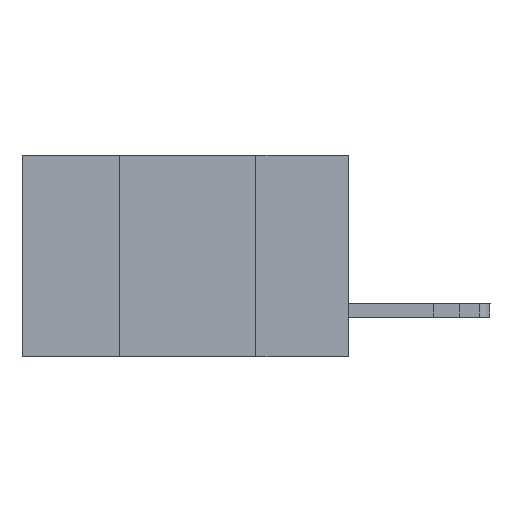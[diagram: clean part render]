
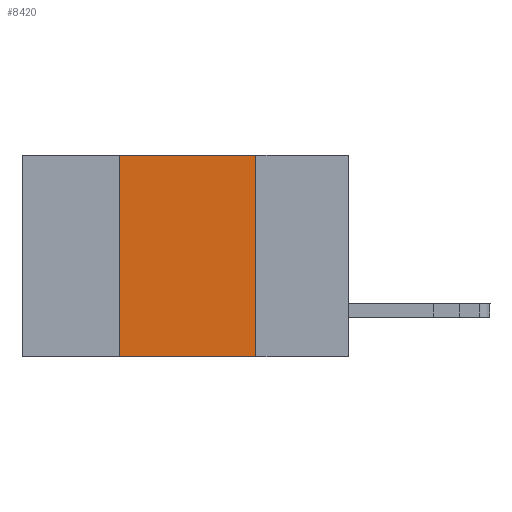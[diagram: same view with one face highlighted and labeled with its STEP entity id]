
A CAD part, left-side view. The second image highlights one B-rep face of the part: STEP entity #8420.
In plain terms, the highlighted planar face has unit normal (-1, 0, 0).
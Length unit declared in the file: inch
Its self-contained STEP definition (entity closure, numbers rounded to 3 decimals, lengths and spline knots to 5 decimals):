
#33 = DIRECTION ( 'NONE',  ( 0., 0., 1. ) ) ;
#223 = ORIENTED_EDGE ( 'NONE', *, *, #5374, .F. ) ;
#313 = CARTESIAN_POINT ( 'NONE',  ( 0., 0.42, -0.37 ) ) ;
#810 = DIRECTION ( 'NONE',  ( 0., -1., 0. ) ) ;
#1038 = CARTESIAN_POINT ( 'NONE',  ( 0., 0.6, 0. ) ) ;
#1165 = CARTESIAN_POINT ( 'NONE',  ( 0., 0.17, 0. ) ) ;
#2223 = VECTOR ( 'NONE', #12008, 39.37008 ) ;
#3703 = LINE ( 'NONE', #313, #11901 ) ;
#4192 = EDGE_CURVE ( 'NONE', #19816, #11647, #16184, .T. ) ;
#4987 = LINE ( 'NONE', #1038, #9142 ) ;
#5374 = EDGE_CURVE ( 'NONE', #19816, #12864, #3703, .T. ) ;
#5771 = FACE_OUTER_BOUND ( 'NONE', #6441, .T. ) ;
#6441 = EDGE_LOOP ( 'NONE', ( #13106, #18326, #223, #18880 ) ) ;
#7774 = EDGE_CURVE ( 'NONE', #12864, #18358, #4987, .T. ) ;
#8179 = VECTOR ( 'NONE', #15052, 39.37008 ) ;
#8420 = ADVANCED_FACE ( 'NONE', ( #5771 ), #18574, .F. ) ;
#8827 = AXIS2_PLACEMENT_3D ( 'NONE', #18517, #18370, #18292 ) ;
#9142 = VECTOR ( 'NONE', #810, 39.37008 ) ;
#11241 = EDGE_CURVE ( 'NONE', #18358, #11647, #22503, .T. ) ;
#11647 = VERTEX_POINT ( 'NONE', #12137 ) ;
#11901 = VECTOR ( 'NONE', #33, 39.37008 ) ;
#12008 = DIRECTION ( 'NONE',  ( 0., -1., 0. ) ) ;
#12041 = CARTESIAN_POINT ( 'NONE',  ( 0., 0.6, -0.37 ) ) ;
#12137 = CARTESIAN_POINT ( 'NONE',  ( 0., 0.17, -0.37 ) ) ;
#12864 = VERTEX_POINT ( 'NONE', #13517 ) ;
#13106 = ORIENTED_EDGE ( 'NONE', *, *, #11241, .F. ) ;
#13517 = CARTESIAN_POINT ( 'NONE',  ( 0., 0.42, 0. ) ) ;
#15052 = DIRECTION ( 'NONE',  ( 0., 0., -1. ) ) ;
#15528 = CARTESIAN_POINT ( 'NONE',  ( 0., 0.17, -0.37 ) ) ;
#16184 = LINE ( 'NONE', #12041, #2223 ) ;
#18292 = DIRECTION ( 'NONE',  ( 0., 0., -1. ) ) ;
#18326 = ORIENTED_EDGE ( 'NONE', *, *, #7774, .F. ) ;
#18358 = VERTEX_POINT ( 'NONE', #1165 ) ;
#18370 = DIRECTION ( 'NONE',  ( 1., 0., 0. ) ) ;
#18517 = CARTESIAN_POINT ( 'NONE',  ( 0., 0.6, 0. ) ) ;
#18574 = PLANE ( 'NONE',  #8827 ) ;
#18880 = ORIENTED_EDGE ( 'NONE', *, *, #4192, .T. ) ;
#19816 = VERTEX_POINT ( 'NONE', #21246 ) ;
#21246 = CARTESIAN_POINT ( 'NONE',  ( 0., 0.42, -0.37 ) ) ;
#22503 = LINE ( 'NONE', #15528, #8179 ) ;
